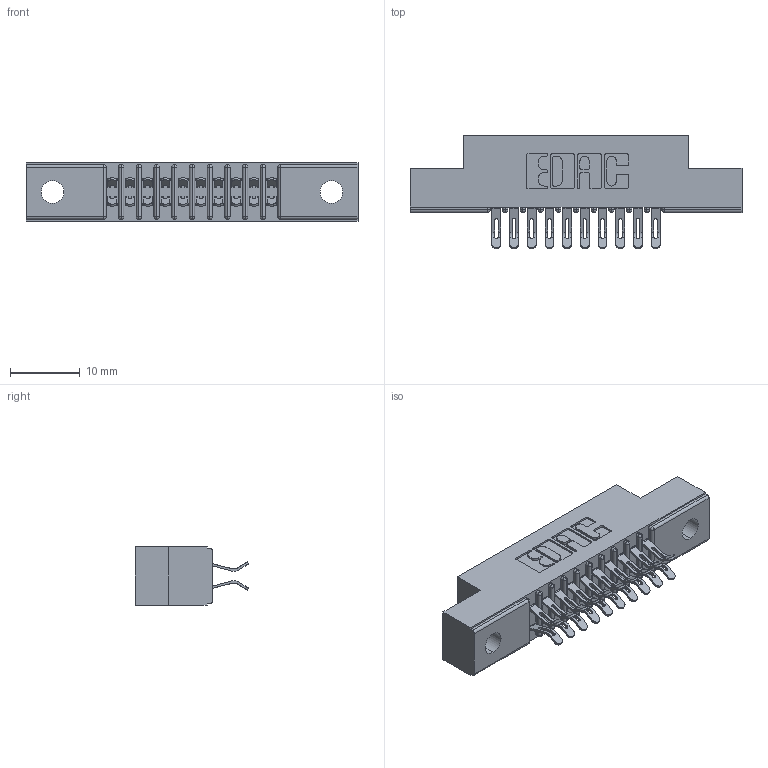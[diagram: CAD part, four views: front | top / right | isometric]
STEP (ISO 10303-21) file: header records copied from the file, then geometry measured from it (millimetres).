
FILE_DESCRIPTION (( 'STEP AP203' ), '1' );
FILE_NAME ('391-020-555-202.STEP', '2018-08-08T18:57:28', ( '' ), ( '' ), 'SwSTEP 2.0', 'SolidWorks 2016', '' );
FILE_SCHEMA (( 'CONFIG_CONTROL_DESIGN' ));
Length unit declared in the file: inch
Products named in the file (3): 341 Part_.128 (3.25) Dia Mounting Holes; 341-292-001_341-292-155; 391-020-555-202
Assembly tree (21 placements, depth 2):
  391-020-555-202
    341 Part_.128 (3.25) Dia Mounting Holes
    341-292-001_341-292-155  x20
Bounding box: 47.62 x 16.31 x 8.38 mm (x, y, z)
Volume: 2729.4 mm3; surface area: 4862.8 mm2
Topology: 21 solids, 21 shells, 1676 faces, 4986 edges, 3246 vertices
Faces by surface type: plane 908, cylinder 728, sphere 22, torus 18
Entity records: 16837 total; most frequent: CARTESIAN_POINT 2816, ORIENTED_EDGE 2784, DIRECTION 2746, EDGE_CURVE 1392, VECTOR 1074, LINE 1074, VERTEX_POINT 890, AXIS2_PLACEMENT_3D 836
